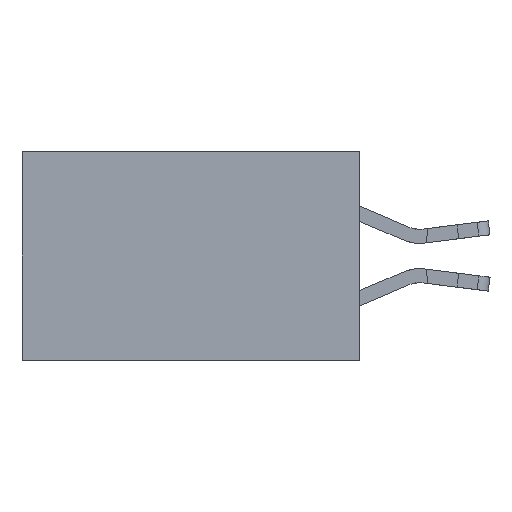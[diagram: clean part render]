
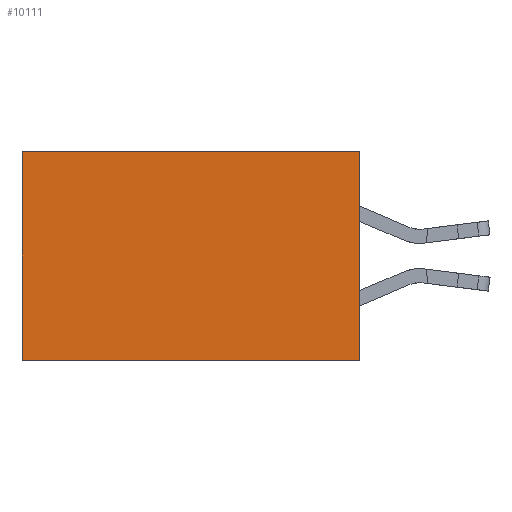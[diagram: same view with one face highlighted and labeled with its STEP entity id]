
A CAD part, left-side view. The second image highlights one B-rep face of the part: STEP entity #10111.
In plain terms, the highlighted planar face has unit normal (-1, 0, 0).
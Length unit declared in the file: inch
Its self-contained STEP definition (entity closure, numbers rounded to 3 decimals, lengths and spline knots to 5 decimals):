
#510 = DIRECTION ( 'NONE',  ( 0., 1., 0. ) ) ;
#589 = ORIENTED_EDGE ( 'NONE', *, *, #6334, .F. ) ;
#763 = VECTOR ( 'NONE', #883, 39.37008 ) ;
#883 = DIRECTION ( 'NONE',  ( 0., 0., -1. ) ) ;
#1796 = AXIS2_PLACEMENT_3D ( 'NONE', #16418, #19334, #7261 ) ;
#2011 = LINE ( 'NONE', #12834, #18939 ) ;
#3686 = VECTOR ( 'NONE', #510, 39.37008 ) ;
#5156 = VERTEX_POINT ( 'NONE', #18217 ) ;
#5673 = CARTESIAN_POINT ( 'NONE',  ( 0.2875, 0.6, 0. ) ) ;
#6097 = ORIENTED_EDGE ( 'NONE', *, *, #6558, .T. ) ;
#6334 = EDGE_CURVE ( 'NONE', #13931, #6389, #12633, .T. ) ;
#6389 = VERTEX_POINT ( 'NONE', #12488 ) ;
#6558 = EDGE_CURVE ( 'NONE', #5156, #6389, #16495, .T. ) ;
#7261 = DIRECTION ( 'NONE',  ( 0., 0., -1. ) ) ;
#8919 = CARTESIAN_POINT ( 'NONE',  ( 0.2875, 0., -0.37 ) ) ;
#8932 = CARTESIAN_POINT ( 'NONE',  ( 0.2875, 0., -0.37 ) ) ;
#9153 = CARTESIAN_POINT ( 'NONE',  ( 0.2875, 0., 0. ) ) ;
#9520 = FACE_OUTER_BOUND ( 'NONE', #16323, .T. ) ;
#10002 = CARTESIAN_POINT ( 'NONE',  ( 0.2875, 0., 0. ) ) ;
#10111 = ADVANCED_FACE ( 'NONE', ( #9520 ), #16205, .F. ) ;
#10529 = DIRECTION ( 'NONE',  ( 0., 1., 0. ) ) ;
#10555 = EDGE_CURVE ( 'NONE', #15076, #13931, #2011, .T. ) ;
#11172 = VECTOR ( 'NONE', #10529, 39.37008 ) ;
#11448 = ORIENTED_EDGE ( 'NONE', *, *, #19451, .T. ) ;
#12401 = LINE ( 'NONE', #10002, #3686 ) ;
#12488 = CARTESIAN_POINT ( 'NONE',  ( 0.2875, 0.6, -0.37 ) ) ;
#12633 = LINE ( 'NONE', #8919, #11172 ) ;
#12834 = CARTESIAN_POINT ( 'NONE',  ( 0.2875, 0., 0. ) ) ;
#13931 = VERTEX_POINT ( 'NONE', #8932 ) ;
#14622 = ORIENTED_EDGE ( 'NONE', *, *, #10555, .F. ) ;
#15076 = VERTEX_POINT ( 'NONE', #9153 ) ;
#16205 = PLANE ( 'NONE',  #1796 ) ;
#16323 = EDGE_LOOP ( 'NONE', ( #6097, #589, #14622, #11448 ) ) ;
#16418 = CARTESIAN_POINT ( 'NONE',  ( 0.2875, 0., 0. ) ) ;
#16495 = LINE ( 'NONE', #5673, #763 ) ;
#18217 = CARTESIAN_POINT ( 'NONE',  ( 0.2875, 0.6, 0. ) ) ;
#18939 = VECTOR ( 'NONE', #19113, 39.37008 ) ;
#19113 = DIRECTION ( 'NONE',  ( 0., 0., -1. ) ) ;
#19334 = DIRECTION ( 'NONE',  ( 1., 0., 0. ) ) ;
#19451 = EDGE_CURVE ( 'NONE', #15076, #5156, #12401, .T. ) ;
